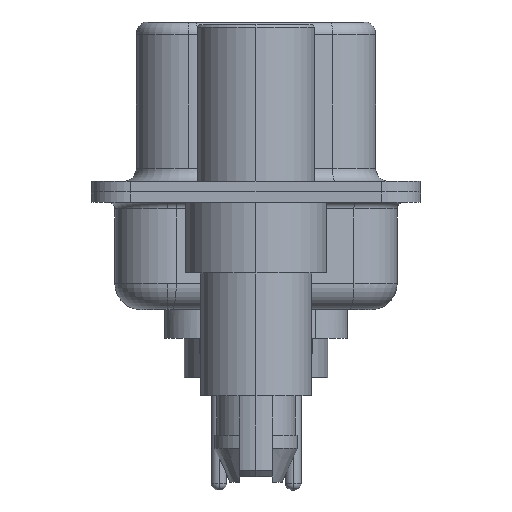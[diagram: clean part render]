
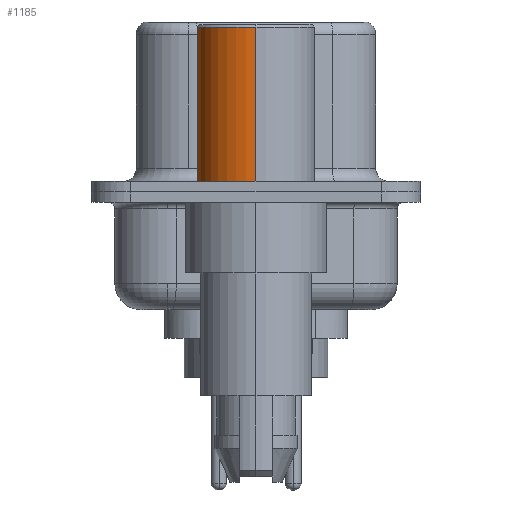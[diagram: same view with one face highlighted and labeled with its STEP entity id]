
A CAD part, left-side view. The second image highlights one B-rep face of the part: STEP entity #1185.
In plain terms, the highlighted cylindrical face has radius 2.25 mm (diameter 4.5 mm), a partial arc.
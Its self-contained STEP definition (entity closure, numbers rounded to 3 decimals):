
#128 = CARTESIAN_POINT ( 'NONE',  ( 2.25, 0., 6.3 ) ) ;
#416 = CARTESIAN_POINT ( 'NONE',  ( -2.25, 0., 0.581 ) ) ;
#486 = LINE ( 'NONE', #416, #14957 ) ;
#603 = ORIENTED_EDGE ( 'NONE', *, *, #11442, .T. ) ;
#1185 = ADVANCED_FACE ( 'NONE', ( #5057 ), #11868, .T. ) ;
#1298 = CARTESIAN_POINT ( 'NONE',  ( 0., 0., 0.581 ) ) ;
#1299 = AXIS2_PLACEMENT_3D ( 'NONE', #13927, #5743, #15325 ) ;
#2721 = LINE ( 'NONE', #12701, #10029 ) ;
#3640 = CARTESIAN_POINT ( 'NONE',  ( -2.25, 0., 6.3 ) ) ;
#4051 = DIRECTION ( 'NONE',  ( 1., 0., 0. ) ) ;
#4115 = ORIENTED_EDGE ( 'NONE', *, *, #11457, .T. ) ;
#5057 = FACE_OUTER_BOUND ( 'NONE', #6160, .T. ) ;
#5201 = ORIENTED_EDGE ( 'NONE', *, *, #11367, .F. ) ;
#5506 = CARTESIAN_POINT ( 'NONE',  ( 0., 0., 6.3 ) ) ;
#5727 = CIRCLE ( 'NONE', #9876, 2.25 ) ;
#5743 = DIRECTION ( 'NONE',  ( 0., 0., 1. ) ) ;
#6160 = EDGE_LOOP ( 'NONE', ( #603, #4115, #5201, #8667 ) ) ;
#6898 = DIRECTION ( 'NONE',  ( 1., 0., 0. ) ) ;
#8280 = CARTESIAN_POINT ( 'NONE',  ( 2.25, 0., 0.4 ) ) ;
#8523 = DIRECTION ( 'NONE',  ( 0., 0., 1. ) ) ;
#8667 = ORIENTED_EDGE ( 'NONE', *, *, #11526, .F. ) ;
#9293 = DIRECTION ( 'NONE',  ( 0., 0., 1. ) ) ;
#9736 = CARTESIAN_POINT ( 'NONE',  ( -2.25, 0., 0.4 ) ) ;
#9876 = AXIS2_PLACEMENT_3D ( 'NONE', #5506, #15096, #6898 ) ;
#9906 = VERTEX_POINT ( 'NONE', #3640 ) ;
#10029 = VECTOR ( 'NONE', #14051, 1000. ) ;
#11366 = VERTEX_POINT ( 'NONE', #128 ) ;
#11367 = EDGE_CURVE ( 'NONE', #11366, #9906, #5727, .T. ) ;
#11442 = EDGE_CURVE ( 'NONE', #12317, #12345, #11676, .T. ) ;
#11457 = EDGE_CURVE ( 'NONE', #12345, #9906, #486, .T. ) ;
#11526 = EDGE_CURVE ( 'NONE', #12317, #11366, #2721, .T. ) ;
#11676 = CIRCLE ( 'NONE', #1299, 2.25 ) ;
#11868 = CYLINDRICAL_SURFACE ( 'NONE', #14606, 2.25 ) ;
#12317 = VERTEX_POINT ( 'NONE', #8280 ) ;
#12345 = VERTEX_POINT ( 'NONE', #9736 ) ;
#12701 = CARTESIAN_POINT ( 'NONE',  ( 2.25, 0., 0.581 ) ) ;
#13927 = CARTESIAN_POINT ( 'NONE',  ( 0., 0., 0.4 ) ) ;
#14051 = DIRECTION ( 'NONE',  ( 0., 0., 1. ) ) ;
#14606 = AXIS2_PLACEMENT_3D ( 'NONE', #1298, #9293, #4051 ) ;
#14957 = VECTOR ( 'NONE', #8523, 1000. ) ;
#15096 = DIRECTION ( 'NONE',  ( 0., 0., 1. ) ) ;
#15325 = DIRECTION ( 'NONE',  ( 1., 0., 0. ) ) ;
